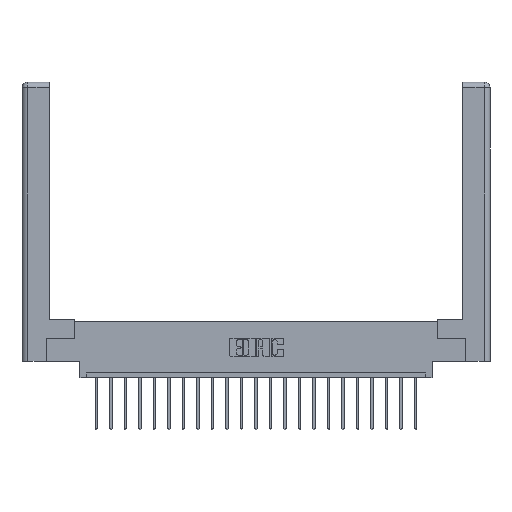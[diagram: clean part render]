
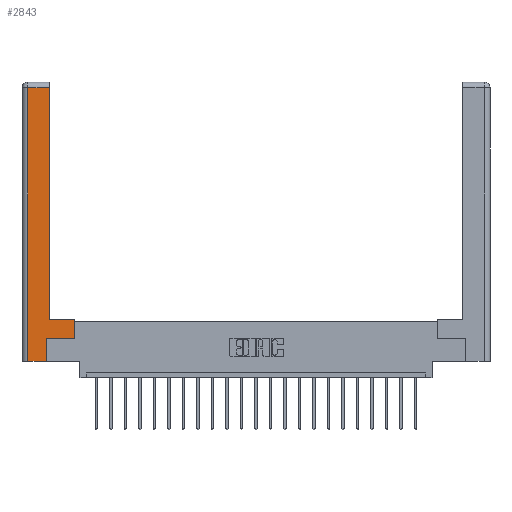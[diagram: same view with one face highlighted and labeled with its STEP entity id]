
A CAD part, top view. The second image highlights one B-rep face of the part: STEP entity #2843.
In plain terms, the highlighted planar face has unit normal (0, 0, 1).
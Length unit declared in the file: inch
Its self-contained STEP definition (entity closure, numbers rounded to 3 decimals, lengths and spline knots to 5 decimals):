
#288 = ORIENTED_EDGE ( 'NONE', *, *, #10539, .T. ) ;
#360 = VECTOR ( 'NONE', #6349, 39.37008 ) ;
#878 = ORIENTED_EDGE ( 'NONE', *, *, #8322, .T. ) ;
#1033 = VERTEX_POINT ( 'NONE', #16965 ) ;
#1100 = VECTOR ( 'NONE', #16378, 39.37008 ) ;
#1178 = ORIENTED_EDGE ( 'NONE', *, *, #11555, .T. ) ;
#1599 = FACE_OUTER_BOUND ( 'NONE', #17776, .T. ) ;
#2172 = VERTEX_POINT ( 'NONE', #3953 ) ;
#2353 = AXIS2_PLACEMENT_3D ( 'NONE', #8683, #8757, #8600 ) ;
#2843 = ADVANCED_FACE ( 'NONE', ( #1599 ), #15677, .F. ) ;
#3251 = CARTESIAN_POINT ( 'NONE',  ( 0.565, 0.45, 0. ) ) ;
#3293 = CARTESIAN_POINT ( 'NONE',  ( 0.265, 0.245, 0. ) ) ;
#3459 = DIRECTION ( 'NONE',  ( 0., 1., 0. ) ) ;
#3622 = VERTEX_POINT ( 'NONE', #18419 ) ;
#3739 = VERTEX_POINT ( 'NONE', #22292 ) ;
#3953 = CARTESIAN_POINT ( 'NONE',  ( 0.295, 0.45, 0. ) ) ;
#3954 = LINE ( 'NONE', #7220, #16126 ) ;
#5007 = ORIENTED_EDGE ( 'NONE', *, *, #15970, .T. ) ;
#5550 = CARTESIAN_POINT ( 'NONE',  ( 0.0615, 0., 0. ) ) ;
#5753 = CARTESIAN_POINT ( 'NONE',  ( 0.265, 0., 0. ) ) ;
#5921 = CARTESIAN_POINT ( 'NONE',  ( 0.565, 0.245, 0. ) ) ;
#6148 = EDGE_CURVE ( 'NONE', #3622, #2172, #3954, .T. ) ;
#6349 = DIRECTION ( 'NONE',  ( 1., 0., 0. ) ) ;
#6597 = ORIENTED_EDGE ( 'NONE', *, *, #13405, .T. ) ;
#7101 = CARTESIAN_POINT ( 'NONE',  ( 0.265, 0., 0. ) ) ;
#7220 = CARTESIAN_POINT ( 'NONE',  ( 0.295, 0.45, 0. ) ) ;
#7593 = LINE ( 'NONE', #5550, #12113 ) ;
#7607 = DIRECTION ( 'NONE',  ( -1., 0., 0. ) ) ;
#8171 = VERTEX_POINT ( 'NONE', #13285 ) ;
#8322 = EDGE_CURVE ( 'NONE', #8376, #15582, #18104, .T. ) ;
#8376 = VERTEX_POINT ( 'NONE', #21088 ) ;
#8600 = DIRECTION ( 'NONE',  ( -1., 0., 0. ) ) ;
#8683 = CARTESIAN_POINT ( 'NONE',  ( 0., 0., 0. ) ) ;
#8757 = DIRECTION ( 'NONE',  ( 0., 0., -1. ) ) ;
#8872 = LINE ( 'NONE', #19468, #21248 ) ;
#8974 = DIRECTION ( 'NONE',  ( 1., 0., 0. ) ) ;
#9393 = LINE ( 'NONE', #3293, #18278 ) ;
#9750 = VERTEX_POINT ( 'NONE', #5921 ) ;
#9982 = VECTOR ( 'NONE', #8974, 39.37008 ) ;
#10001 = ORIENTED_EDGE ( 'NONE', *, *, #6148, .T. ) ;
#10539 = EDGE_CURVE ( 'NONE', #15582, #3739, #9393, .T. ) ;
#11555 = EDGE_CURVE ( 'NONE', #3739, #9750, #19273, .T. ) ;
#11813 = DIRECTION ( 'NONE',  ( 0., 1., 0. ) ) ;
#12113 = VECTOR ( 'NONE', #21035, 39.37008 ) ;
#12201 = LINE ( 'NONE', #3251, #14908 ) ;
#13011 = LINE ( 'NONE', #19680, #1100 ) ;
#13285 = CARTESIAN_POINT ( 'NONE',  ( 0.295, 2.94, 0. ) ) ;
#13405 = EDGE_CURVE ( 'NONE', #8171, #1033, #8872, .T. ) ;
#14256 = DIRECTION ( 'NONE',  ( -1., 0., 0. ) ) ;
#14908 = VECTOR ( 'NONE', #11813, 39.37008 ) ;
#15582 = VERTEX_POINT ( 'NONE', #7101 ) ;
#15677 = PLANE ( 'NONE',  #2353 ) ;
#15970 = EDGE_CURVE ( 'NONE', #9750, #3622, #12201, .T. ) ;
#16126 = VECTOR ( 'NONE', #7607, 39.37008 ) ;
#16378 = DIRECTION ( 'NONE',  ( 0., 1., 0. ) ) ;
#16898 = CARTESIAN_POINT ( 'NONE',  ( 0.565, 0.245, 0. ) ) ;
#16965 = CARTESIAN_POINT ( 'NONE',  ( 0.0615, 2.94, 0. ) ) ;
#17776 = EDGE_LOOP ( 'NONE', ( #20411, #6597, #22002, #878, #288, #1178, #5007, #10001 ) ) ;
#17781 = EDGE_CURVE ( 'NONE', #1033, #8376, #7593, .T. ) ;
#18104 = LINE ( 'NONE', #5753, #9982 ) ;
#18278 = VECTOR ( 'NONE', #3459, 39.37008 ) ;
#18419 = CARTESIAN_POINT ( 'NONE',  ( 0.565, 0.45, 0. ) ) ;
#19273 = LINE ( 'NONE', #16898, #360 ) ;
#19468 = CARTESIAN_POINT ( 'NONE',  ( 0.0615, 2.94, 0. ) ) ;
#19680 = CARTESIAN_POINT ( 'NONE',  ( 0.295, 3., 0. ) ) ;
#19864 = EDGE_CURVE ( 'NONE', #2172, #8171, #13011, .T. ) ;
#20411 = ORIENTED_EDGE ( 'NONE', *, *, #19864, .T. ) ;
#21035 = DIRECTION ( 'NONE',  ( 0., -1., 0. ) ) ;
#21088 = CARTESIAN_POINT ( 'NONE',  ( 0.0615, 0., 0. ) ) ;
#21248 = VECTOR ( 'NONE', #14256, 39.37008 ) ;
#22002 = ORIENTED_EDGE ( 'NONE', *, *, #17781, .T. ) ;
#22292 = CARTESIAN_POINT ( 'NONE',  ( 0.265, 0.245, 0. ) ) ;
